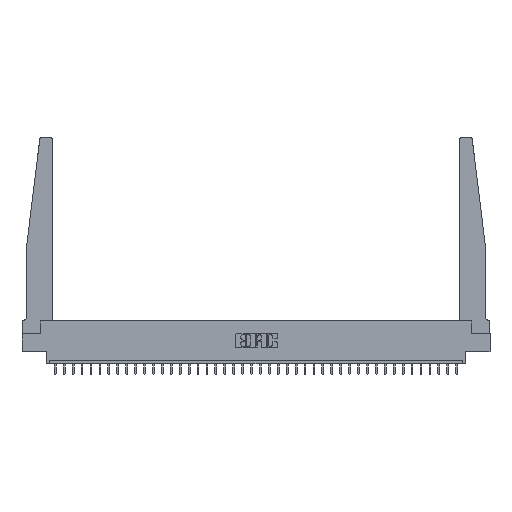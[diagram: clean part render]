
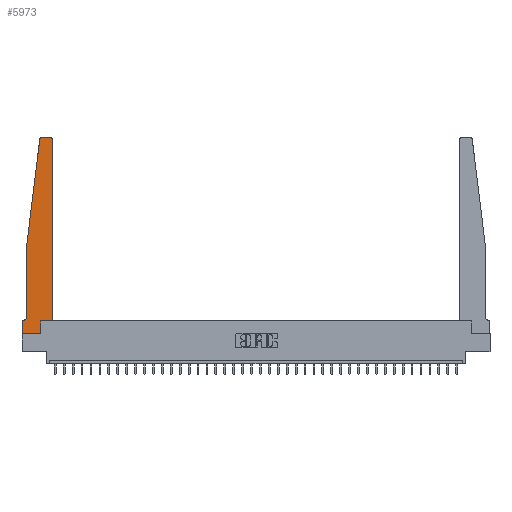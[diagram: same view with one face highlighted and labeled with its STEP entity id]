
A CAD part, top view. The second image highlights one B-rep face of the part: STEP entity #5973.
In plain terms, the highlighted planar face has unit normal (0, 0, 1).
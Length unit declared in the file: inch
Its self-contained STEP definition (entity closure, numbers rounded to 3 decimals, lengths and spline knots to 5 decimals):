
#4 = VERTEX_POINT ( 'NONE', #25904 ) ;
#140 = VECTOR ( 'NONE', #3805, 39.37008 ) ;
#180 = VERTEX_POINT ( 'NONE', #13933 ) ;
#498 = FACE_OUTER_BOUND ( 'NONE', #19582, .T. ) ;
#721 = VERTEX_POINT ( 'NONE', #2753 ) ;
#1251 = VECTOR ( 'NONE', #23652, 39.37008 ) ;
#1549 = ORIENTED_EDGE ( 'NONE', *, *, #24011, .T. ) ;
#1927 = CARTESIAN_POINT ( 'NONE',  ( 0.015, 0.2375, 0.37 ) ) ;
#1935 = CARTESIAN_POINT ( 'NONE',  ( 0.25, 2.75, 0.37 ) ) ;
#2417 = DIRECTION ( 'NONE',  ( 1., 0., 0. ) ) ;
#2440 = CARTESIAN_POINT ( 'NONE',  ( 0., 0., 0.37 ) ) ;
#2684 = EDGE_CURVE ( 'NONE', #6170, #4, #25563, .T. ) ;
#2753 = CARTESIAN_POINT ( 'NONE',  ( 0.425, 2.72, 0.37 ) ) ;
#3026 = VECTOR ( 'NONE', #24051, 39.37008 ) ;
#3208 = CARTESIAN_POINT ( 'NONE',  ( 0., 0.1875, 0.37 ) ) ;
#3237 = CIRCLE ( 'NONE', #19409, 0.03 ) ;
#3469 = CARTESIAN_POINT ( 'NONE',  ( 0.425, 0.18, 0.37 ) ) ;
#3534 = LINE ( 'NONE', #24773, #30093 ) ;
#3580 = CARTESIAN_POINT ( 'NONE',  ( 0.24675, 2.72367, 0.37 ) ) ;
#3805 = DIRECTION ( 'NONE',  ( -1., 0., 0. ) ) ;
#4768 = CARTESIAN_POINT ( 'NONE',  ( 0.27653, 2.72, 0.37 ) ) ;
#4972 = DIRECTION ( 'NONE',  ( 0., 0., 1. ) ) ;
#5076 = DIRECTION ( 'NONE',  ( 0., 1., 0. ) ) ;
#5369 = ORIENTED_EDGE ( 'NONE', *, *, #16243, .T. ) ;
#5973 = ADVANCED_FACE ( 'NONE', ( #498 ), #28859, .T. ) ;
#6170 = VERTEX_POINT ( 'NONE', #33156 ) ;
#6213 = DIRECTION ( 'NONE',  ( -1., 0., 0. ) ) ;
#6363 = ORIENTED_EDGE ( 'NONE', *, *, #28150, .T. ) ;
#6550 = VERTEX_POINT ( 'NONE', #8943 ) ;
#6765 = ORIENTED_EDGE ( 'NONE', *, *, #28955, .T. ) ;
#7303 = ORIENTED_EDGE ( 'NONE', *, *, #15663, .T. ) ;
#8647 = DIRECTION ( 'NONE',  ( -0.122, -0.992, 0. ) ) ;
#8943 = CARTESIAN_POINT ( 'NONE',  ( 0.27653, 2.75, 0.37 ) ) ;
#9387 = VECTOR ( 'NONE', #5076, 39.37008 ) ;
#9795 = AXIS2_PLACEMENT_3D ( 'NONE', #1927, #9858, #6213 ) ;
#9828 = CARTESIAN_POINT ( 'NONE',  ( 0.065, 1.25, 0.37 ) ) ;
#9858 = DIRECTION ( 'NONE',  ( 0., 0., -1. ) ) ;
#10035 = DIRECTION ( 'NONE',  ( 1., 0., 0. ) ) ;
#10063 = EDGE_CURVE ( 'NONE', #17709, #25794, #25841, .T. ) ;
#10164 = ORIENTED_EDGE ( 'NONE', *, *, #11149, .T. ) ;
#10510 = LINE ( 'NONE', #29054, #1251 ) ;
#10710 = DIRECTION ( 'NONE',  ( 1., 0., 0. ) ) ;
#10743 = VECTOR ( 'NONE', #10710, 39.37008 ) ;
#11149 = EDGE_CURVE ( 'NONE', #721, #16866, #3237, .T. ) ;
#11518 = CIRCLE ( 'NONE', #30354, 0.03 ) ;
#12207 = DIRECTION ( 'NONE',  ( 0., 0., 1. ) ) ;
#12333 = EDGE_CURVE ( 'NONE', #4, #18152, #20499, .T. ) ;
#12579 = DIRECTION ( 'NONE',  ( 0., -1., 0. ) ) ;
#12620 = VERTEX_POINT ( 'NONE', #22343 ) ;
#13015 = CARTESIAN_POINT ( 'NONE',  ( 0.2605, 0.18, 0.37 ) ) ;
#13933 = CARTESIAN_POINT ( 'NONE',  ( 0.2605, 0., 0.37 ) ) ;
#15138 = VERTEX_POINT ( 'NONE', #23824 ) ;
#15513 = CARTESIAN_POINT ( 'NONE',  ( 0.395, 2.75, 0.37 ) ) ;
#15663 = EDGE_CURVE ( 'NONE', #16866, #6550, #19328, .T. ) ;
#16041 = LINE ( 'NONE', #13015, #9387 ) ;
#16243 = EDGE_CURVE ( 'NONE', #6550, #17709, #11518, .T. ) ;
#16368 = EDGE_CURVE ( 'NONE', #12620, #721, #10510, .T. ) ;
#16866 = VERTEX_POINT ( 'NONE', #15513 ) ;
#17709 = VERTEX_POINT ( 'NONE', #3580 ) ;
#18152 = VERTEX_POINT ( 'NONE', #27149 ) ;
#18272 = VECTOR ( 'NONE', #8647, 39.37008 ) ;
#18743 = DIRECTION ( 'NONE',  ( 0., 0., 1. ) ) ;
#19103 = EDGE_CURVE ( 'NONE', #180, #15138, #16041, .T. ) ;
#19216 = DIRECTION ( 'NONE',  ( 0., -1., 0. ) ) ;
#19328 = LINE ( 'NONE', #1935, #140 ) ;
#19375 = VECTOR ( 'NONE', #12579, 39.37008 ) ;
#19409 = AXIS2_PLACEMENT_3D ( 'NONE', #30953, #4972, #10035 ) ;
#19582 = EDGE_LOOP ( 'NONE', ( #7303, #5369, #31855, #6363, #21130, #25989, #24167, #6765, #22203, #1549, #20146, #10164 ) ) ;
#20146 = ORIENTED_EDGE ( 'NONE', *, *, #16368, .T. ) ;
#20165 = DIRECTION ( 'NONE',  ( -1., 0., 0. ) ) ;
#20499 = LINE ( 'NONE', #23193, #19375 ) ;
#20659 = AXIS2_PLACEMENT_3D ( 'NONE', #3208, #18743, #2417 ) ;
#21130 = ORIENTED_EDGE ( 'NONE', *, *, #31493, .T. ) ;
#22203 = ORIENTED_EDGE ( 'NONE', *, *, #19103, .T. ) ;
#22343 = CARTESIAN_POINT ( 'NONE',  ( 0.425, 0.18, 0.37 ) ) ;
#23193 = CARTESIAN_POINT ( 'NONE',  ( 0., 0., 0.37 ) ) ;
#23652 = DIRECTION ( 'NONE',  ( 0., 1., 0. ) ) ;
#23824 = CARTESIAN_POINT ( 'NONE',  ( 0.2605, 0.18, 0.37 ) ) ;
#24011 = EDGE_CURVE ( 'NONE', #15138, #12620, #29443, .T. ) ;
#24051 = DIRECTION ( 'NONE',  ( 1., 0., 0. ) ) ;
#24167 = ORIENTED_EDGE ( 'NONE', *, *, #12333, .T. ) ;
#24355 = CIRCLE ( 'NONE', #9795, 0.05 ) ;
#24773 = CARTESIAN_POINT ( 'NONE',  ( 0.065, 1.25, 0.37 ) ) ;
#25563 = LINE ( 'NONE', #32994, #28759 ) ;
#25794 = VERTEX_POINT ( 'NONE', #9828 ) ;
#25841 = LINE ( 'NONE', #29712, #18272 ) ;
#25904 = CARTESIAN_POINT ( 'NONE',  ( 0., 0.1875, 0.37 ) ) ;
#25989 = ORIENTED_EDGE ( 'NONE', *, *, #2684, .T. ) ;
#27149 = CARTESIAN_POINT ( 'NONE',  ( 0., 0., 0.37 ) ) ;
#27649 = VERTEX_POINT ( 'NONE', #31583 ) ;
#28150 = EDGE_CURVE ( 'NONE', #25794, #27649, #3534, .T. ) ;
#28422 = LINE ( 'NONE', #2440, #10743 ) ;
#28759 = VECTOR ( 'NONE', #20165, 39.37008 ) ;
#28859 = PLANE ( 'NONE',  #20659 ) ;
#28955 = EDGE_CURVE ( 'NONE', #18152, #180, #28422, .T. ) ;
#29054 = CARTESIAN_POINT ( 'NONE',  ( 0.425, 0.18, 0.37 ) ) ;
#29443 = LINE ( 'NONE', #3469, #3026 ) ;
#29712 = CARTESIAN_POINT ( 'NONE',  ( 0.065, 1.25, 0.37 ) ) ;
#30093 = VECTOR ( 'NONE', #19216, 39.37008 ) ;
#30354 = AXIS2_PLACEMENT_3D ( 'NONE', #4768, #12207, #30574 ) ;
#30574 = DIRECTION ( 'NONE',  ( 1., 0., 0. ) ) ;
#30953 = CARTESIAN_POINT ( 'NONE',  ( 0.395, 2.72, 0.37 ) ) ;
#31493 = EDGE_CURVE ( 'NONE', #27649, #6170, #24355, .T. ) ;
#31583 = CARTESIAN_POINT ( 'NONE',  ( 0.065, 0.2375, 0.37 ) ) ;
#31855 = ORIENTED_EDGE ( 'NONE', *, *, #10063, .T. ) ;
#32994 = CARTESIAN_POINT ( 'NONE',  ( 0.065, 0.1875, 0.37 ) ) ;
#33156 = CARTESIAN_POINT ( 'NONE',  ( 0.015, 0.1875, 0.37 ) ) ;
